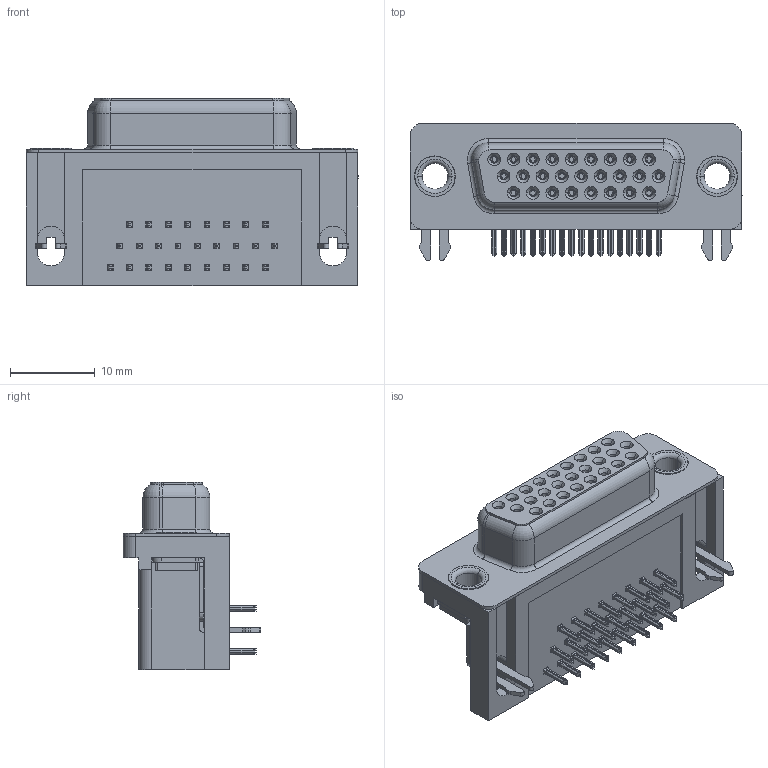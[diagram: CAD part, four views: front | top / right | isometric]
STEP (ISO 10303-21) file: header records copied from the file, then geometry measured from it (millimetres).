
FILE_DESCRIPTION (( 'STEP AP203' ), '1' );
FILE_NAME ('634-026-363-531.STEP', '2018-08-18T03:30:56', ( '' ), ( '' ), 'SwSTEP 2.0', 'SolidWorks 2016', '' );
FILE_SCHEMA (( 'CONFIG_CONTROL_DESIGN' ));
Length unit declared in the file: millimetre
Products named in the file (8): 2 Prong Board Lock; Thru Hole Rivet; 634-026-363-531; 634 Housing_26 Socket; 634 Shell_26 Socket; Contact Bottom; Contact Middle; Contact Top
Assembly tree (32 placements, depth 2):
  634-026-363-531
    634 Housing_26 Socket
    634 Shell_26 Socket
    Contact Bottom  x8
    Contact Middle  x9
    Contact Top  x9
    2 Prong Board Lock  x2
    Thru Hole Rivet  x2
Bounding box: 39.22 x 16.25 x 22.1 mm (x, y, z)
Volume: 6353.8 mm3; surface area: 9065.2 mm2
Topology: 32 solids, 32 shells, 3981 faces, 10474 edges, 6582 vertices
Faces by surface type: plane 1803, cylinder 928, bspline 904, cone 312, torus 34
Entity records: 35116 total; most frequent: CARTESIAN_POINT 10512, ORIENTED_EDGE 4970, DIRECTION 4429, EDGE_CURVE 2485, LINE 1615, VECTOR 1615, VERTEX_POINT 1584, AXIS2_PLACEMENT_3D 1407
